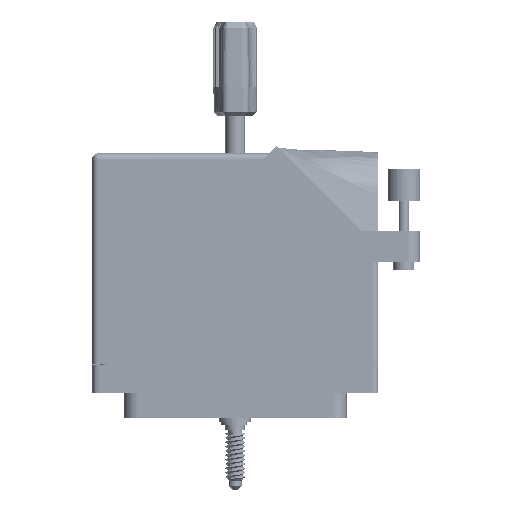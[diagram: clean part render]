
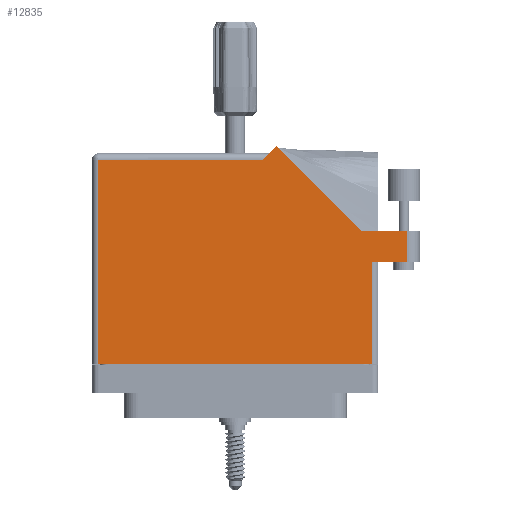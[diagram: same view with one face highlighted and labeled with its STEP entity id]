
A CAD part, front view. The second image highlights one B-rep face of the part: STEP entity #12835.
In plain terms, the highlighted face is planar.
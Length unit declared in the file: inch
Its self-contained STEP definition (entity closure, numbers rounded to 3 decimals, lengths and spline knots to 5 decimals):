
#297 = LINE ( 'NONE', #76862, #24659 ) ;
#463 = PLANE ( 'NONE',  #54856 ) ;
#1021 = VECTOR ( 'NONE', #22997, 39.37008 ) ;
#1695 = CARTESIAN_POINT ( 'NONE',  ( 0.39821, 2.00071, 0.765 ) ) ;
#2023 = CARTESIAN_POINT ( 'NONE',  ( -1.3155, -0.1, 0.765 ) ) ;
#2729 = DIRECTION ( 'NONE',  ( -0.707, 0.707, 0. ) ) ;
#2800 = CARTESIAN_POINT ( 'NONE',  ( -1.3775, 1.868, 0.765 ) ) ;
#4534 = DIRECTION ( 'NONE',  ( -1., 0., 0. ) ) ;
#5820 = DIRECTION ( 'NONE',  ( 1., 0., 0. ) ) ;
#8994 = CARTESIAN_POINT ( 'NONE',  ( -1.3775, 1.93, 0.765 ) ) ;
#9345 = DIRECTION ( 'NONE',  ( -1., 0., 0. ) ) ;
#10209 = EDGE_CURVE ( 'NONE', #48677, #54110, #41817, .T. ) ;
#12835 = ADVANCED_FACE ( 'NONE', ( #45294 ), #463, .F. ) ;
#13136 = CARTESIAN_POINT ( 'NONE',  ( 1.6525, 1.187, 0.765 ) ) ;
#15406 = EDGE_CURVE ( 'NONE', #51408, #36318, #17931, .T. ) ;
#15947 = ORIENTED_EDGE ( 'NONE', *, *, #10209, .T. ) ;
#17167 = ORIENTED_EDGE ( 'NONE', *, *, #15406, .T. ) ;
#17931 = LINE ( 'NONE', #51193, #36010 ) ;
#19095 = DIRECTION ( 'NONE',  ( 0., 1., 0. ) ) ;
#21703 = EDGE_CURVE ( 'NONE', #41385, #51408, #91311, .T. ) ;
#22010 = CARTESIAN_POINT ( 'NONE',  ( 1.3155, -0.1, 0.765 ) ) ;
#22997 = DIRECTION ( 'NONE',  ( 1., 0., 0. ) ) ;
#23684 = VECTOR ( 'NONE', #2729, 39.37008 ) ;
#24380 = DIRECTION ( 'NONE',  ( -1., 0., 0. ) ) ;
#24659 = VECTOR ( 'NONE', #19095, 39.37008 ) ;
#26289 = DIRECTION ( 'NONE',  ( 0., 1., 0. ) ) ;
#32794 = CARTESIAN_POINT ( 'NONE',  ( 1.3155, 0.88, 0.765 ) ) ;
#32993 = EDGE_CURVE ( 'NONE', #70243, #41385, #49057, .T. ) ;
#34878 = EDGE_CURVE ( 'NONE', #36318, #48677, #75467, .T. ) ;
#36010 = VECTOR ( 'NONE', #92641, 39.37008 ) ;
#36318 = VERTEX_POINT ( 'NONE', #47282 ) ;
#38174 = LINE ( 'NONE', #55450, #1021 ) ;
#40719 = VERTEX_POINT ( 'NONE', #32794 ) ;
#41385 = VERTEX_POINT ( 'NONE', #88481 ) ;
#41817 = LINE ( 'NONE', #50880, #46923 ) ;
#45230 = ORIENTED_EDGE ( 'NONE', *, *, #32993, .T. ) ;
#45294 = FACE_OUTER_BOUND ( 'NONE', #69644, .T. ) ;
#45863 = CARTESIAN_POINT ( 'NONE',  ( 1.3775, 0.88, 0.765 ) ) ;
#46619 = VECTOR ( 'NONE', #26289, 39.37008 ) ;
#46923 = VECTOR ( 'NONE', #83780, 39.37008 ) ;
#47282 = CARTESIAN_POINT ( 'NONE',  ( 0.2655, 1.868, 0.765 ) ) ;
#48611 = CARTESIAN_POINT ( 'NONE',  ( 1.7775, 1.187, 0.765 ) ) ;
#48677 = VERTEX_POINT ( 'NONE', #57466 ) ;
#49057 = LINE ( 'NONE', #48611, #105303 ) ;
#50880 = CARTESIAN_POINT ( 'NONE',  ( -1.3155, -0.1, 0.765 ) ) ;
#51159 = CARTESIAN_POINT ( 'NONE',  ( 1.6525, 0.88, 0.765 ) ) ;
#51193 = CARTESIAN_POINT ( 'NONE',  ( 0.3275, 1.93, 0.765 ) ) ;
#51408 = VERTEX_POINT ( 'NONE', #1695 ) ;
#54110 = VERTEX_POINT ( 'NONE', #2023 ) ;
#54674 = ORIENTED_EDGE ( 'NONE', *, *, #34878, .T. ) ;
#54856 = AXIS2_PLACEMENT_3D ( 'NONE', #8994, #58320, #9345 ) ;
#55450 = CARTESIAN_POINT ( 'NONE',  ( -1.3775, -0.1, 0.765 ) ) ;
#57466 = CARTESIAN_POINT ( 'NONE',  ( -1.3155, 1.868, 0.765 ) ) ;
#58013 = CARTESIAN_POINT ( 'NONE',  ( 1.6525, 1.187, 0.765 ) ) ;
#58076 = ORIENTED_EDGE ( 'NONE', *, *, #104432, .T. ) ;
#58320 = DIRECTION ( 'NONE',  ( 0., 0., -1. ) ) ;
#58471 = VECTOR ( 'NONE', #5820, 39.37008 ) ;
#61041 = LINE ( 'NONE', #45863, #58471 ) ;
#63956 = ORIENTED_EDGE ( 'NONE', *, *, #21703, .T. ) ;
#64073 = ORIENTED_EDGE ( 'NONE', *, *, #97545, .T. ) ;
#68926 = VERTEX_POINT ( 'NONE', #22010 ) ;
#69644 = EDGE_LOOP ( 'NONE', ( #100849, #64073, #45230, #63956, #17167, #54674, #15947, #58076, #102242 ) ) ;
#69656 = LINE ( 'NONE', #58013, #46619 ) ;
#70243 = VERTEX_POINT ( 'NONE', #13136 ) ;
#75467 = LINE ( 'NONE', #2800, #99761 ) ;
#75944 = CARTESIAN_POINT ( 'NONE',  ( 1.21192, 1.187, 0.765 ) ) ;
#76862 = CARTESIAN_POINT ( 'NONE',  ( 1.3155, 0.88, 0.765 ) ) ;
#79468 = VERTEX_POINT ( 'NONE', #51159 ) ;
#83780 = DIRECTION ( 'NONE',  ( 0., -1., 0. ) ) ;
#86896 = EDGE_CURVE ( 'NONE', #68926, #40719, #297, .T. ) ;
#88481 = CARTESIAN_POINT ( 'NONE',  ( 1.21192, 1.187, 0.765 ) ) ;
#91311 = LINE ( 'NONE', #75944, #23684 ) ;
#92641 = DIRECTION ( 'NONE',  ( -0.707, -0.707, 0. ) ) ;
#94735 = EDGE_CURVE ( 'NONE', #40719, #79468, #61041, .T. ) ;
#97545 = EDGE_CURVE ( 'NONE', #79468, #70243, #69656, .T. ) ;
#99761 = VECTOR ( 'NONE', #4534, 39.37008 ) ;
#100849 = ORIENTED_EDGE ( 'NONE', *, *, #94735, .T. ) ;
#102242 = ORIENTED_EDGE ( 'NONE', *, *, #86896, .T. ) ;
#104432 = EDGE_CURVE ( 'NONE', #54110, #68926, #38174, .T. ) ;
#105303 = VECTOR ( 'NONE', #24380, 39.37008 ) ;
